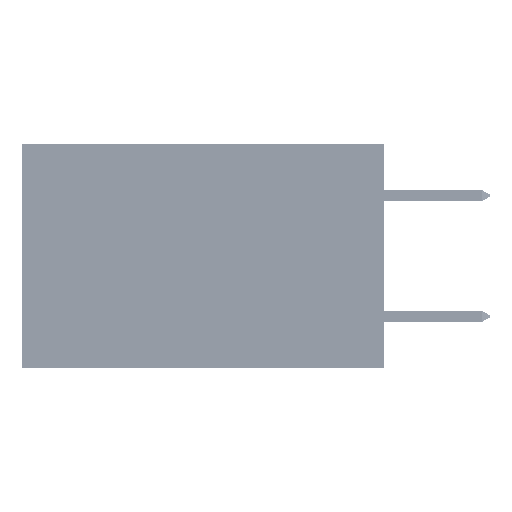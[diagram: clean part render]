
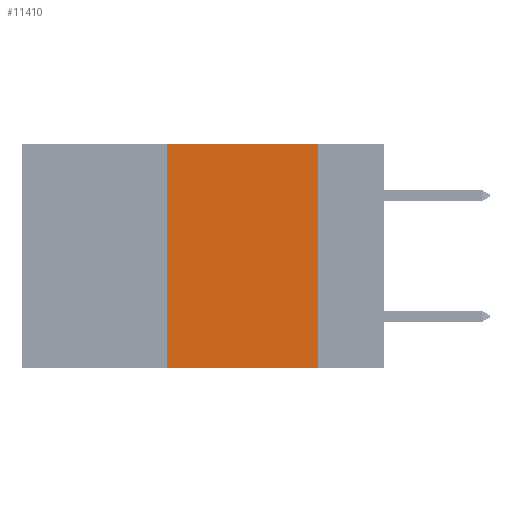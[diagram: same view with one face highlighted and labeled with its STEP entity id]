
A CAD part, left-side view. The second image highlights one B-rep face of the part: STEP entity #11410.
In plain terms, the highlighted planar face has unit normal (-1, 0, 0).
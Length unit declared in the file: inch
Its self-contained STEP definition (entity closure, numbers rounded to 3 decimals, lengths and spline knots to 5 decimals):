
#89 = LINE ( 'NONE', #4924, #2511 ) ;
#884 = ORIENTED_EDGE ( 'NONE', *, *, #15368, .T. ) ;
#1047 = LINE ( 'NONE', #30998, #36811 ) ;
#2511 = VECTOR ( 'NONE', #43360, 39.37008 ) ;
#2825 = VERTEX_POINT ( 'NONE', #17603 ) ;
#3633 = EDGE_CURVE ( 'NONE', #14693, #29293, #48471, .T. ) ;
#4444 = CARTESIAN_POINT ( 'NONE',  ( 0., 0.6, 0. ) ) ;
#4924 = CARTESIAN_POINT ( 'NONE',  ( 0., 0.6, -0.37 ) ) ;
#6916 = ORIENTED_EDGE ( 'NONE', *, *, #3633, .F. ) ;
#11410 = ADVANCED_FACE ( 'NONE', ( #28315 ), #46455, .F. ) ;
#11603 = DIRECTION ( 'NONE',  ( 0., -1., 0. ) ) ;
#14693 = VERTEX_POINT ( 'NONE', #15330 ) ;
#14894 = AXIS2_PLACEMENT_3D ( 'NONE', #4444, #19455, #27290 ) ;
#14993 = CARTESIAN_POINT ( 'NONE',  ( 0., 0.36, -0.37 ) ) ;
#15330 = CARTESIAN_POINT ( 'NONE',  ( 0., 0.36, 0. ) ) ;
#15368 = EDGE_CURVE ( 'NONE', #34005, #2825, #89, .T. ) ;
#17603 = CARTESIAN_POINT ( 'NONE',  ( 0., 0.11, -0.37 ) ) ;
#19455 = DIRECTION ( 'NONE',  ( 1., 0., 0. ) ) ;
#19702 = EDGE_CURVE ( 'NONE', #29293, #2825, #1047, .T. ) ;
#19926 = VECTOR ( 'NONE', #39604, 39.37008 ) ;
#20031 = CARTESIAN_POINT ( 'NONE',  ( 0., 0.6, 0. ) ) ;
#23706 = EDGE_LOOP ( 'NONE', ( #28286, #6916, #43780, #884 ) ) ;
#24349 = CARTESIAN_POINT ( 'NONE',  ( 0., 0.36, 0. ) ) ;
#27290 = DIRECTION ( 'NONE',  ( 0., 0., -1. ) ) ;
#28286 = ORIENTED_EDGE ( 'NONE', *, *, #19702, .F. ) ;
#28315 = FACE_OUTER_BOUND ( 'NONE', #23706, .T. ) ;
#28619 = CARTESIAN_POINT ( 'NONE',  ( 0., 0.11, 0. ) ) ;
#29293 = VERTEX_POINT ( 'NONE', #28619 ) ;
#30998 = CARTESIAN_POINT ( 'NONE',  ( 0., 0.11, 0. ) ) ;
#31490 = LINE ( 'NONE', #24349, #19926 ) ;
#34005 = VERTEX_POINT ( 'NONE', #14993 ) ;
#36420 = EDGE_CURVE ( 'NONE', #34005, #14693, #31490, .T. ) ;
#36811 = VECTOR ( 'NONE', #46445, 39.37008 ) ;
#39604 = DIRECTION ( 'NONE',  ( 0., 0., 1. ) ) ;
#43360 = DIRECTION ( 'NONE',  ( 0., -1., 0. ) ) ;
#43780 = ORIENTED_EDGE ( 'NONE', *, *, #36420, .F. ) ;
#46445 = DIRECTION ( 'NONE',  ( 0., 0., -1. ) ) ;
#46455 = PLANE ( 'NONE',  #14894 ) ;
#48471 = LINE ( 'NONE', #20031, #49049 ) ;
#49049 = VECTOR ( 'NONE', #11603, 39.37008 ) ;
